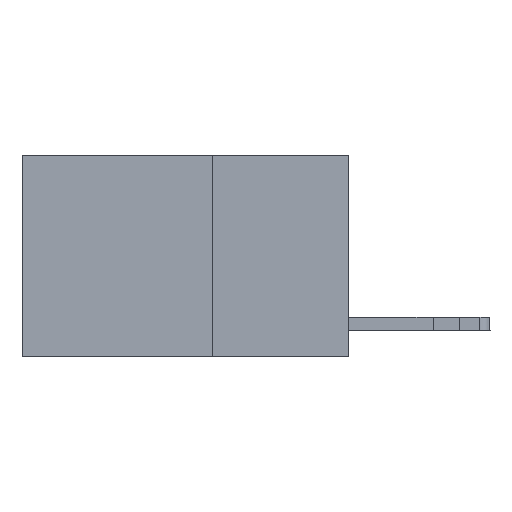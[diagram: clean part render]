
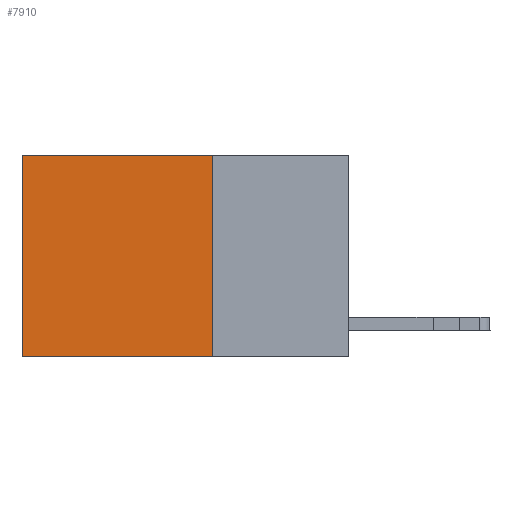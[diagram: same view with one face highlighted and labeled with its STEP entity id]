
A CAD part, left-side view. The second image highlights one B-rep face of the part: STEP entity #7910.
In plain terms, the highlighted planar face has unit normal (-1, 0, 0).
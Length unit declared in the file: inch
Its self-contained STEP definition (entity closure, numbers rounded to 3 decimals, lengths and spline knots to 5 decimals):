
#49 = CARTESIAN_POINT ( 'NONE',  ( 0.2625, 0.25, 0. ) ) ;
#102 = VERTEX_POINT ( 'NONE', #10208 ) ;
#1625 = VECTOR ( 'NONE', #8510, 39.37008 ) ;
#1908 = EDGE_LOOP ( 'NONE', ( #4534, #7918, #10288, #2459 ) ) ;
#2459 = ORIENTED_EDGE ( 'NONE', *, *, #7433, .T. ) ;
#2567 = DIRECTION ( 'NONE',  ( 0., 0., -1. ) ) ;
#2740 = PLANE ( 'NONE',  #8101 ) ;
#4517 = VERTEX_POINT ( 'NONE', #4567 ) ;
#4534 = ORIENTED_EDGE ( 'NONE', *, *, #7642, .T. ) ;
#4549 = VECTOR ( 'NONE', #5757, 39.37008 ) ;
#4567 = CARTESIAN_POINT ( 'NONE',  ( 0.2625, 0.25, -0.37 ) ) ;
#5232 = DIRECTION ( 'NONE',  ( 0., 0., -1. ) ) ;
#5367 = VECTOR ( 'NONE', #8740, 39.37008 ) ;
#5757 = DIRECTION ( 'NONE',  ( 0., 1., 0. ) ) ;
#6425 = CARTESIAN_POINT ( 'NONE',  ( 0.2625, 0.25, 0. ) ) ;
#7032 = CARTESIAN_POINT ( 'NONE',  ( 0.2625, 0.25, 0. ) ) ;
#7433 = EDGE_CURVE ( 'NONE', #14368, #102, #15957, .T. ) ;
#7642 = EDGE_CURVE ( 'NONE', #102, #12472, #12602, .T. ) ;
#7715 = CARTESIAN_POINT ( 'NONE',  ( 0.2625, 0.25, 0. ) ) ;
#7910 = ADVANCED_FACE ( 'NONE', ( #10531 ), #2740, .F. ) ;
#7918 = ORIENTED_EDGE ( 'NONE', *, *, #11976, .F. ) ;
#8101 = AXIS2_PLACEMENT_3D ( 'NONE', #49, #16999, #2567 ) ;
#8510 = DIRECTION ( 'NONE',  ( 0., 1., 0. ) ) ;
#8665 = CARTESIAN_POINT ( 'NONE',  ( 0.2625, 0.6, -0.37 ) ) ;
#8740 = DIRECTION ( 'NONE',  ( 0., 0., -1. ) ) ;
#9935 = CARTESIAN_POINT ( 'NONE',  ( 0.2625, 0.6, 0. ) ) ;
#10208 = CARTESIAN_POINT ( 'NONE',  ( 0.2625, 0.6, 0. ) ) ;
#10288 = ORIENTED_EDGE ( 'NONE', *, *, #13189, .F. ) ;
#10531 = FACE_OUTER_BOUND ( 'NONE', #1908, .T. ) ;
#10652 = VECTOR ( 'NONE', #5232, 39.37008 ) ;
#11976 = EDGE_CURVE ( 'NONE', #4517, #12472, #13914, .T. ) ;
#12472 = VERTEX_POINT ( 'NONE', #8665 ) ;
#12602 = LINE ( 'NONE', #9935, #5367 ) ;
#13189 = EDGE_CURVE ( 'NONE', #14368, #4517, #14230, .T. ) ;
#13914 = LINE ( 'NONE', #15121, #1625 ) ;
#14230 = LINE ( 'NONE', #7715, #10652 ) ;
#14368 = VERTEX_POINT ( 'NONE', #6425 ) ;
#15121 = CARTESIAN_POINT ( 'NONE',  ( 0.2625, 0.25, -0.37 ) ) ;
#15957 = LINE ( 'NONE', #7032, #4549 ) ;
#16999 = DIRECTION ( 'NONE',  ( 1., 0., 0. ) ) ;
